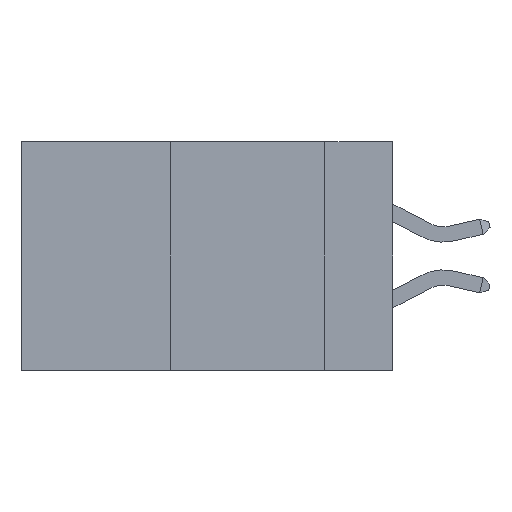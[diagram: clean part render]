
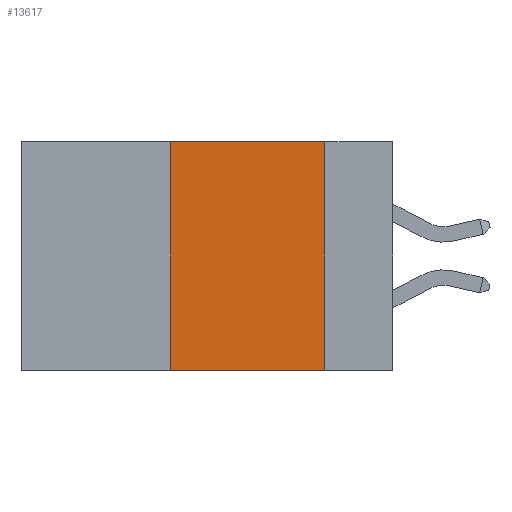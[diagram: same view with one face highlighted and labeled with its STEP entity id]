
A CAD part, left-side view. The second image highlights one B-rep face of the part: STEP entity #13617.
In plain terms, the highlighted planar face has unit normal (-1, 0, 0).
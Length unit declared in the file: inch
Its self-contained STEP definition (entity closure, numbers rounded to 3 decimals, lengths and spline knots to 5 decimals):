
#923 = DIRECTION ( 'NONE',  ( 0., 0., -1. ) ) ;
#1461 = EDGE_CURVE ( 'NONE', #10695, #23700, #26759, .T. ) ;
#1582 = VECTOR ( 'NONE', #6534, 39.37008 ) ;
#1770 = ORIENTED_EDGE ( 'NONE', *, *, #1461, .F. ) ;
#2207 = FACE_OUTER_BOUND ( 'NONE', #14221, .T. ) ;
#5893 = DIRECTION ( 'NONE',  ( 1., 0., 0. ) ) ;
#6534 = DIRECTION ( 'NONE',  ( 0., -1., 0. ) ) ;
#7858 = VECTOR ( 'NONE', #11141, 39.37008 ) ;
#8356 = VERTEX_POINT ( 'NONE', #21807 ) ;
#10284 = VECTOR ( 'NONE', #923, 39.37008 ) ;
#10695 = VERTEX_POINT ( 'NONE', #24077 ) ;
#11141 = DIRECTION ( 'NONE',  ( 0., -1., 0. ) ) ;
#11787 = CARTESIAN_POINT ( 'NONE',  ( 0., 0.11, 0. ) ) ;
#11825 = CARTESIAN_POINT ( 'NONE',  ( 0., 0.36, 0. ) ) ;
#13617 = ADVANCED_FACE ( 'NONE', ( #2207 ), #21435, .F. ) ;
#14221 = EDGE_LOOP ( 'NONE', ( #1770, #18503, #14726, #21620 ) ) ;
#14444 = CARTESIAN_POINT ( 'NONE',  ( 0., 0.36, 0. ) ) ;
#14726 = ORIENTED_EDGE ( 'NONE', *, *, #24372, .F. ) ;
#15028 = EDGE_CURVE ( 'NONE', #8356, #23700, #25893, .T. ) ;
#16952 = CARTESIAN_POINT ( 'NONE',  ( 0., 0.6, 0. ) ) ;
#18503 = ORIENTED_EDGE ( 'NONE', *, *, #20969, .F. ) ;
#18952 = LINE ( 'NONE', #14444, #23406 ) ;
#19352 = LINE ( 'NONE', #16952, #7858 ) ;
#20969 = EDGE_CURVE ( 'NONE', #24599, #10695, #19352, .T. ) ;
#21208 = DIRECTION ( 'NONE',  ( 0., 0., 1. ) ) ;
#21255 = CARTESIAN_POINT ( 'NONE',  ( 0., 0.6, -0.37 ) ) ;
#21435 = PLANE ( 'NONE',  #23165 ) ;
#21620 = ORIENTED_EDGE ( 'NONE', *, *, #15028, .T. ) ;
#21807 = CARTESIAN_POINT ( 'NONE',  ( 0., 0.36, -0.37 ) ) ;
#23165 = AXIS2_PLACEMENT_3D ( 'NONE', #27649, #5893, #25503 ) ;
#23406 = VECTOR ( 'NONE', #21208, 39.37008 ) ;
#23700 = VERTEX_POINT ( 'NONE', #24767 ) ;
#24077 = CARTESIAN_POINT ( 'NONE',  ( 0., 0.11, 0. ) ) ;
#24372 = EDGE_CURVE ( 'NONE', #8356, #24599, #18952, .T. ) ;
#24599 = VERTEX_POINT ( 'NONE', #11825 ) ;
#24767 = CARTESIAN_POINT ( 'NONE',  ( 0., 0.11, -0.37 ) ) ;
#25503 = DIRECTION ( 'NONE',  ( 0., 0., -1. ) ) ;
#25893 = LINE ( 'NONE', #21255, #1582 ) ;
#26759 = LINE ( 'NONE', #11787, #10284 ) ;
#27649 = CARTESIAN_POINT ( 'NONE',  ( 0., 0.6, 0. ) ) ;
